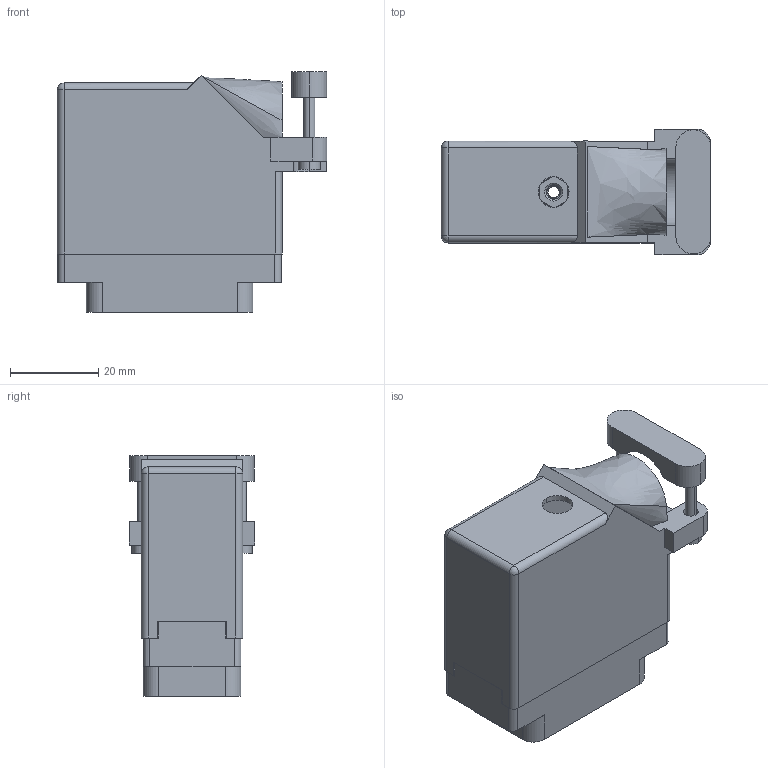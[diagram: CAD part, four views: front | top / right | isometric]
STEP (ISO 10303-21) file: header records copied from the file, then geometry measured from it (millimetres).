
FILE_DESCRIPTION (( 'STEP AP203' ), '1' );
FILE_NAME ('516-038-000-546.STEP', '2020-03-09T18:58:52', ( '' ), ( '' ), 'SwSTEP 2.0', 'SolidWorks 2016', '' );
FILE_SCHEMA (( 'CONFIG_CONTROL_DESIGN' ));
Length unit declared in the file: inch
Products named in the file (4): 516-252-035-100_516-252-035-100; 516-038-000-546; 516 Plug Insulator_038; 516-230-001_Plastic - 038 Side Entry - Large Clamp
Assembly tree (3 placements, depth 2):
  516-038-000-546
    516 Plug Insulator_038
    516-230-001_Plastic - 038 Side Entry - Large Clamp
    516-252-035-100_516-252-035-100
Bounding box: 61.21 x 28.57 x 54.69 mm (x, y, z)
Volume: 19799.7 mm3; surface area: 26158.4 mm2
Topology: 3 solids, 3 shells, 1020 faces, 2956 edges, 1964 vertices
Faces by surface type: plane 697, cylinder 300, cone 12, bspline 9, sphere 2
Entity records: 36551 total; most frequent: CARTESIAN_POINT 8483, ORIENTED_EDGE 5908, DIRECTION 5673, EDGE_CURVE 2954, LINE 2161, VECTOR 2161, VERTEX_POINT 1964, AXIS2_PLACEMENT_3D 1756
